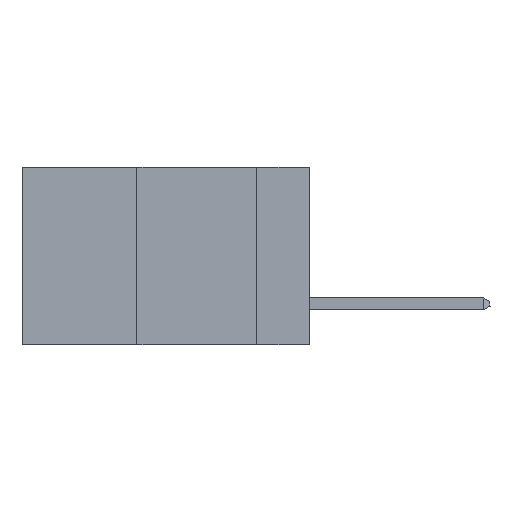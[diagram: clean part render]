
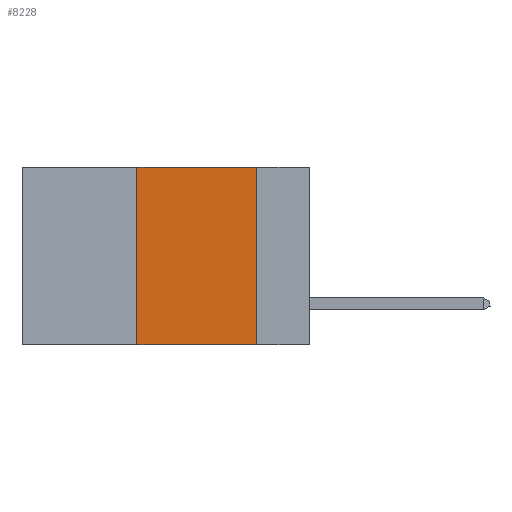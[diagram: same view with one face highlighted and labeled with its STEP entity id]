
A CAD part, left-side view. The second image highlights one B-rep face of the part: STEP entity #8228.
In plain terms, the highlighted planar face has unit normal (-1, 0, 0).
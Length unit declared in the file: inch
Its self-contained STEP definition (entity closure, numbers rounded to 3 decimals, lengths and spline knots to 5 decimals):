
#495 = LINE ( 'NONE', #4342, #19756 ) ;
#532 = DIRECTION ( 'NONE',  ( 1., 0., 0. ) ) ;
#1732 = CARTESIAN_POINT ( 'NONE',  ( 0., 0.11, -0.37 ) ) ;
#1769 = CARTESIAN_POINT ( 'NONE',  ( 0., 0.11, 0. ) ) ;
#2161 = CARTESIAN_POINT ( 'NONE',  ( 0., 0.6, 0. ) ) ;
#3719 = FACE_OUTER_BOUND ( 'NONE', #6882, .T. ) ;
#3844 = VECTOR ( 'NONE', #11875, 39.37008 ) ;
#3921 = ORIENTED_EDGE ( 'NONE', *, *, #11485, .F. ) ;
#3930 = CARTESIAN_POINT ( 'NONE',  ( 0., 0.6, 0. ) ) ;
#4129 = LINE ( 'NONE', #2161, #9681 ) ;
#4342 = CARTESIAN_POINT ( 'NONE',  ( 0., 0.36, 0. ) ) ;
#5162 = VERTEX_POINT ( 'NONE', #1732 ) ;
#6834 = CARTESIAN_POINT ( 'NONE',  ( 0., 0.11, 0. ) ) ;
#6882 = EDGE_LOOP ( 'NONE', ( #3921, #18871, #15919, #17239 ) ) ;
#7428 = DIRECTION ( 'NONE',  ( 0., 0., -1. ) ) ;
#8228 = ADVANCED_FACE ( 'NONE', ( #3719 ), #15932, .F. ) ;
#8240 = CARTESIAN_POINT ( 'NONE',  ( 0., 0.36, -0.37 ) ) ;
#8368 = EDGE_CURVE ( 'NONE', #15040, #5162, #13776, .T. ) ;
#8755 = VERTEX_POINT ( 'NONE', #11451 ) ;
#8818 = EDGE_CURVE ( 'NONE', #15040, #8755, #495, .T. ) ;
#9681 = VECTOR ( 'NONE', #12089, 39.37008 ) ;
#11451 = CARTESIAN_POINT ( 'NONE',  ( 0., 0.36, 0. ) ) ;
#11485 = EDGE_CURVE ( 'NONE', #12169, #5162, #13131, .T. ) ;
#11555 = EDGE_CURVE ( 'NONE', #8755, #12169, #4129, .T. ) ;
#11875 = DIRECTION ( 'NONE',  ( 0., 0., -1. ) ) ;
#12089 = DIRECTION ( 'NONE',  ( 0., -1., 0. ) ) ;
#12169 = VERTEX_POINT ( 'NONE', #1769 ) ;
#13131 = LINE ( 'NONE', #6834, #3844 ) ;
#13776 = LINE ( 'NONE', #16745, #14843 ) ;
#14843 = VECTOR ( 'NONE', #18333, 39.37008 ) ;
#15040 = VERTEX_POINT ( 'NONE', #8240 ) ;
#15919 = ORIENTED_EDGE ( 'NONE', *, *, #8818, .F. ) ;
#15932 = PLANE ( 'NONE',  #19890 ) ;
#16745 = CARTESIAN_POINT ( 'NONE',  ( 0., 0.6, -0.37 ) ) ;
#17239 = ORIENTED_EDGE ( 'NONE', *, *, #8368, .T. ) ;
#18333 = DIRECTION ( 'NONE',  ( 0., -1., 0. ) ) ;
#18871 = ORIENTED_EDGE ( 'NONE', *, *, #11555, .F. ) ;
#19654 = DIRECTION ( 'NONE',  ( 0., 0., 1. ) ) ;
#19756 = VECTOR ( 'NONE', #19654, 39.37008 ) ;
#19890 = AXIS2_PLACEMENT_3D ( 'NONE', #3930, #532, #7428 ) ;
